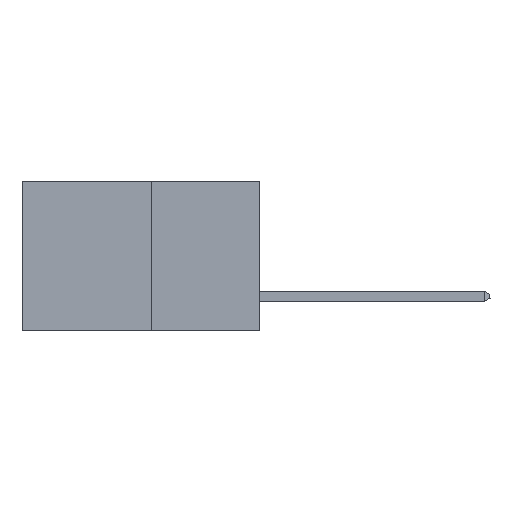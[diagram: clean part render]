
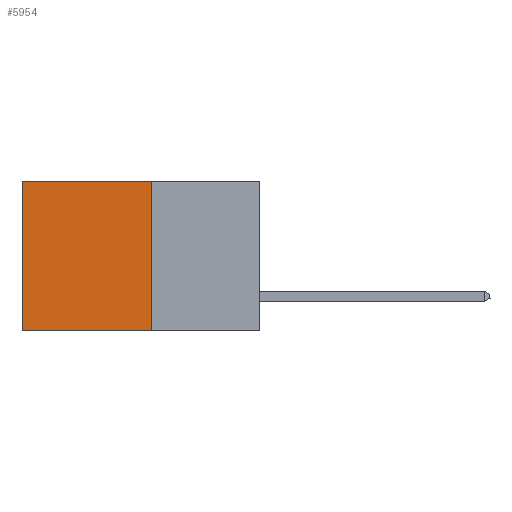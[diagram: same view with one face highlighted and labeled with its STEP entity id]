
A CAD part, left-side view. The second image highlights one B-rep face of the part: STEP entity #5954.
In plain terms, the highlighted planar face has unit normal (-1, 0, 0).
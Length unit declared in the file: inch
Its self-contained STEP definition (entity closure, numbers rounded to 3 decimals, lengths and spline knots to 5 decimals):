
#1063 = LINE ( 'NONE', #21563, #12449 ) ;
#1332 = LINE ( 'NONE', #4136, #25489 ) ;
#1923 = CARTESIAN_POINT ( 'NONE',  ( 0.277, 0.27, -0.37 ) ) ;
#2291 = CARTESIAN_POINT ( 'NONE',  ( 0.277, 0.27, -0.37 ) ) ;
#3068 = EDGE_CURVE ( 'NONE', #16021, #18990, #1332, .T. ) ;
#4136 = CARTESIAN_POINT ( 'NONE',  ( 0.277, 0.59, -0.37 ) ) ;
#5954 = ADVANCED_FACE ( 'NONE', ( #14037 ), #14550, .F. ) ;
#6611 = ORIENTED_EDGE ( 'NONE', *, *, #21964, .F. ) ;
#7440 = EDGE_CURVE ( 'NONE', #27127, #18990, #21220, .T. ) ;
#8005 = CARTESIAN_POINT ( 'NONE',  ( 0.277, 0.27, -0.37 ) ) ;
#10097 = ORIENTED_EDGE ( 'NONE', *, *, #16904, .T. ) ;
#11570 = VERTEX_POINT ( 'NONE', #22667 ) ;
#12066 = ORIENTED_EDGE ( 'NONE', *, *, #3068, .T. ) ;
#12449 = VECTOR ( 'NONE', #30924, 39.37008 ) ;
#14037 = FACE_OUTER_BOUND ( 'NONE', #21365, .T. ) ;
#14509 = DIRECTION ( 'NONE',  ( 0., 0., -1. ) ) ;
#14520 = DIRECTION ( 'NONE',  ( 1., 0., 0. ) ) ;
#14550 = PLANE ( 'NONE',  #28928 ) ;
#14578 = CARTESIAN_POINT ( 'NONE',  ( 0.277, 0.59, -0.37 ) ) ;
#14745 = CARTESIAN_POINT ( 'NONE',  ( 0.277, 0.27, -0.37 ) ) ;
#15240 = DIRECTION ( 'NONE',  ( 0., 0., -1. ) ) ;
#15424 = DIRECTION ( 'NONE',  ( 0., 0., -1. ) ) ;
#16021 = VERTEX_POINT ( 'NONE', #18040 ) ;
#16904 = EDGE_CURVE ( 'NONE', #11570, #16021, #1063, .T. ) ;
#18040 = CARTESIAN_POINT ( 'NONE',  ( 0.277, 0.59, 0. ) ) ;
#18990 = VERTEX_POINT ( 'NONE', #14578 ) ;
#21220 = LINE ( 'NONE', #2291, #26762 ) ;
#21365 = EDGE_LOOP ( 'NONE', ( #12066, #29904, #6611, #10097 ) ) ;
#21563 = CARTESIAN_POINT ( 'NONE',  ( 0.277, 0.27, 0. ) ) ;
#21677 = DIRECTION ( 'NONE',  ( 0., 1., 0. ) ) ;
#21964 = EDGE_CURVE ( 'NONE', #11570, #27127, #30231, .T. ) ;
#22667 = CARTESIAN_POINT ( 'NONE',  ( 0.277, 0.27, 0. ) ) ;
#25489 = VECTOR ( 'NONE', #15424, 39.37008 ) ;
#26762 = VECTOR ( 'NONE', #21677, 39.37008 ) ;
#27127 = VERTEX_POINT ( 'NONE', #1923 ) ;
#28928 = AXIS2_PLACEMENT_3D ( 'NONE', #14745, #14520, #14509 ) ;
#29534 = VECTOR ( 'NONE', #15240, 39.37008 ) ;
#29904 = ORIENTED_EDGE ( 'NONE', *, *, #7440, .F. ) ;
#30231 = LINE ( 'NONE', #8005, #29534 ) ;
#30924 = DIRECTION ( 'NONE',  ( 0., 1., 0. ) ) ;
